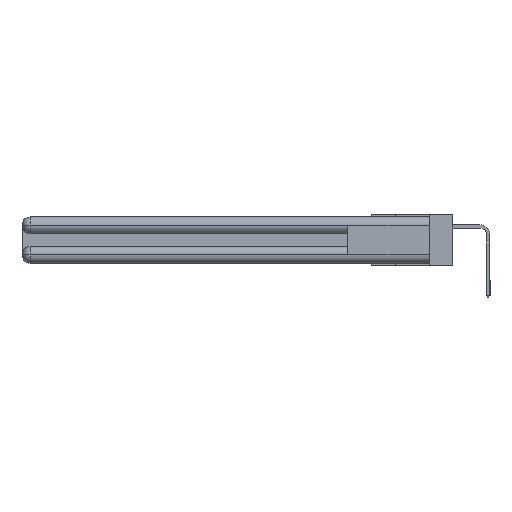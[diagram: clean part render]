
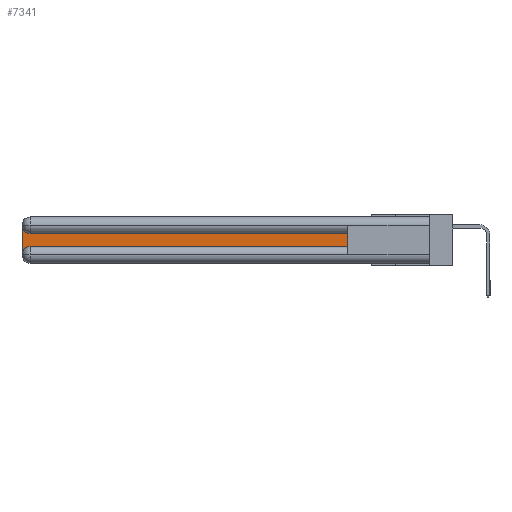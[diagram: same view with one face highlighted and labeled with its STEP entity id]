
A CAD part, left-side view. The second image highlights one B-rep face of the part: STEP entity #7341.
In plain terms, the highlighted planar face has unit normal (-1, 0, 0).
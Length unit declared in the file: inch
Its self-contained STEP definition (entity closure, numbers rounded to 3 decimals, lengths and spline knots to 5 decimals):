
#537 = VECTOR ( 'NONE', #6287, 39.37008 ) ;
#1466 = VERTEX_POINT ( 'NONE', #14360 ) ;
#1579 = CARTESIAN_POINT ( 'NONE',  ( 0.075, 2.94, -0.2775 ) ) ;
#3057 = CARTESIAN_POINT ( 'NONE',  ( 0.075, 0.6, -0.2175 ) ) ;
#3364 = CARTESIAN_POINT ( 'NONE',  ( 0.075, 3., -0.1225 ) ) ;
#4499 = ORIENTED_EDGE ( 'NONE', *, *, #27777, .T. ) ;
#4912 = CARTESIAN_POINT ( 'NONE',  ( 0.075, 0.6, -0.1225 ) ) ;
#5906 = DIRECTION ( 'NONE',  ( 1., 0., 0. ) ) ;
#5957 = EDGE_CURVE ( 'NONE', #8267, #7822, #31831, .T. ) ;
#6287 = DIRECTION ( 'NONE',  ( 0., 0., 1. ) ) ;
#7341 = ADVANCED_FACE ( 'NONE', ( #11220 ), #8430, .F. ) ;
#7351 = ORIENTED_EDGE ( 'NONE', *, *, #5957, .T. ) ;
#7676 = DIRECTION ( 'NONE',  ( 0., 1., 0. ) ) ;
#7822 = VERTEX_POINT ( 'NONE', #17504 ) ;
#8267 = VERTEX_POINT ( 'NONE', #24524 ) ;
#8430 = PLANE ( 'NONE',  #10204 ) ;
#9136 = AXIS2_PLACEMENT_3D ( 'NONE', #33417, #28313, #10054 ) ;
#10054 = DIRECTION ( 'NONE',  ( 0., 0., -1. ) ) ;
#10204 = AXIS2_PLACEMENT_3D ( 'NONE', #3364, #5906, #13689 ) ;
#10367 = CARTESIAN_POINT ( 'NONE',  ( 0.075, 0.6, -0.2175 ) ) ;
#11220 = FACE_OUTER_BOUND ( 'NONE', #30779, .T. ) ;
#13182 = VERTEX_POINT ( 'NONE', #10367 ) ;
#13689 = DIRECTION ( 'NONE',  ( 0., 0., -1. ) ) ;
#14065 = EDGE_CURVE ( 'NONE', #7822, #13182, #30927, .T. ) ;
#14360 = CARTESIAN_POINT ( 'NONE',  ( 0.075, 0.6, -0.1225 ) ) ;
#16441 = CARTESIAN_POINT ( 'NONE',  ( 0.075, 2.94, -0.1225 ) ) ;
#16823 = EDGE_CURVE ( 'NONE', #19810, #23897, #31928, .T. ) ;
#17504 = CARTESIAN_POINT ( 'NONE',  ( 0.075, 2.94, -0.2175 ) ) ;
#19810 = VERTEX_POINT ( 'NONE', #16441 ) ;
#19984 = DIRECTION ( 'NONE',  ( 0., 0., -1. ) ) ;
#20081 = LINE ( 'NONE', #28487, #22166 ) ;
#20680 = LINE ( 'NONE', #3057, #537 ) ;
#21874 = VECTOR ( 'NONE', #28792, 39.37008 ) ;
#22166 = VECTOR ( 'NONE', #33472, 39.37008 ) ;
#22305 = DIRECTION ( 'NONE',  ( 1., 0., 0. ) ) ;
#23072 = CARTESIAN_POINT ( 'NONE',  ( 0.075, 0.6, -0.2175 ) ) ;
#23097 = ORIENTED_EDGE ( 'NONE', *, *, #14065, .T. ) ;
#23855 = AXIS2_PLACEMENT_3D ( 'NONE', #1579, #22305, #19984 ) ;
#23897 = VERTEX_POINT ( 'NONE', #27943 ) ;
#23967 = ORIENTED_EDGE ( 'NONE', *, *, #27484, .T. ) ;
#24524 = CARTESIAN_POINT ( 'NONE',  ( 0.075, 3., -0.2775 ) ) ;
#24614 = LINE ( 'NONE', #4912, #25037 ) ;
#25037 = VECTOR ( 'NONE', #7676, 39.37008 ) ;
#27006 = ORIENTED_EDGE ( 'NONE', *, *, #31133, .T. ) ;
#27202 = ORIENTED_EDGE ( 'NONE', *, *, #16823, .T. ) ;
#27484 = EDGE_CURVE ( 'NONE', #1466, #19810, #24614, .T. ) ;
#27777 = EDGE_CURVE ( 'NONE', #23897, #8267, #20081, .T. ) ;
#27943 = CARTESIAN_POINT ( 'NONE',  ( 0.075, 3., -0.0625 ) ) ;
#28313 = DIRECTION ( 'NONE',  ( 1., 0., 0. ) ) ;
#28487 = CARTESIAN_POINT ( 'NONE',  ( 0.075, 3., -0.2175 ) ) ;
#28792 = DIRECTION ( 'NONE',  ( 0., -1., 0. ) ) ;
#30779 = EDGE_LOOP ( 'NONE', ( #23967, #27202, #4499, #7351, #23097, #27006 ) ) ;
#30927 = LINE ( 'NONE', #23072, #21874 ) ;
#31133 = EDGE_CURVE ( 'NONE', #13182, #1466, #20680, .T. ) ;
#31831 = CIRCLE ( 'NONE', #23855, 0.06 ) ;
#31928 = CIRCLE ( 'NONE', #9136, 0.06 ) ;
#33417 = CARTESIAN_POINT ( 'NONE',  ( 0.075, 2.94, -0.0625 ) ) ;
#33472 = DIRECTION ( 'NONE',  ( 0., 0., -1. ) ) ;
